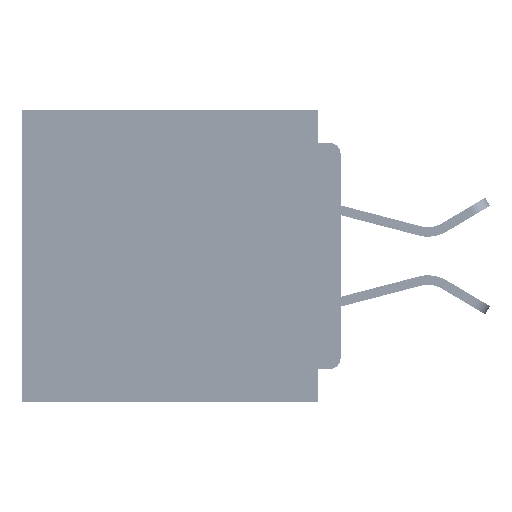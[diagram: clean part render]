
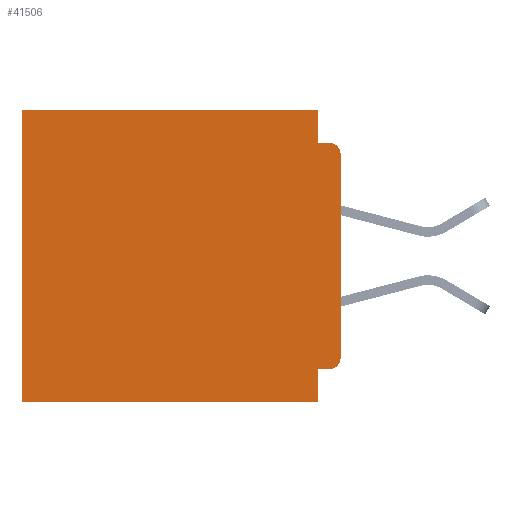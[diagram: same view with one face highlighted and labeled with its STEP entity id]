
A CAD part, left-side view. The second image highlights one B-rep face of the part: STEP entity #41506.
In plain terms, the highlighted planar face has unit normal (-1, 0, 0).
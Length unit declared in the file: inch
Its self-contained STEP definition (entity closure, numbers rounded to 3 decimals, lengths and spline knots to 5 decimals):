
#575 = CARTESIAN_POINT ( 'NONE',  ( 0.3, 0.015, -0.045 ) ) ;
#591 = DIRECTION ( 'NONE',  ( 0., 0., -1. ) ) ;
#2597 = EDGE_CURVE ( 'NONE', #43844, #50518, #33708, .T. ) ;
#2896 = LINE ( 'NONE', #24604, #13809 ) ;
#2907 = ORIENTED_EDGE ( 'NONE', *, *, #11951, .T. ) ;
#3120 = VECTOR ( 'NONE', #52583, 39.37008 ) ;
#3672 = ORIENTED_EDGE ( 'NONE', *, *, #30332, .F. ) ;
#3992 = CARTESIAN_POINT ( 'NONE',  ( 0.3, 0.015, -0.34 ) ) ;
#4407 = VERTEX_POINT ( 'NONE', #10277 ) ;
#4500 = CARTESIAN_POINT ( 'NONE',  ( 0.3, 0.015, -0.355 ) ) ;
#5869 = CARTESIAN_POINT ( 'NONE',  ( 0.3, 0., -0.34 ) ) ;
#5871 = EDGE_CURVE ( 'NONE', #4407, #50518, #24624, .T. ) ;
#6820 = AXIS2_PLACEMENT_3D ( 'NONE', #37404, #9763, #42036 ) ;
#6990 = CARTESIAN_POINT ( 'NONE',  ( 0.3, 0.031, -0.045 ) ) ;
#7002 = CARTESIAN_POINT ( 'NONE',  ( 0.3, 0.437, -0.4 ) ) ;
#7388 = PLANE ( 'NONE',  #40994 ) ;
#8461 = EDGE_CURVE ( 'NONE', #45742, #45604, #2896, .T. ) ;
#8656 = DIRECTION ( 'NONE',  ( 0., 0., -1. ) ) ;
#9176 = VECTOR ( 'NONE', #16141, 39.37008 ) ;
#9763 = DIRECTION ( 'NONE',  ( -1., 0., 0. ) ) ;
#10277 = CARTESIAN_POINT ( 'NONE',  ( 0.3, 0., -0.06 ) ) ;
#10694 = DIRECTION ( 'NONE',  ( 0., 1., 0. ) ) ;
#11133 = EDGE_CURVE ( 'NONE', #12591, #52123, #28607, .T. ) ;
#11951 = EDGE_CURVE ( 'NONE', #32054, #45604, #17674, .T. ) ;
#12055 = DIRECTION ( 'NONE',  ( 1., 0., 0. ) ) ;
#12591 = VERTEX_POINT ( 'NONE', #4500 ) ;
#13768 = LINE ( 'NONE', #38740, #3120 ) ;
#13809 = VECTOR ( 'NONE', #10694, 39.37008 ) ;
#14869 = ORIENTED_EDGE ( 'NONE', *, *, #21734, .F. ) ;
#16141 = DIRECTION ( 'NONE',  ( 0., -1., 0. ) ) ;
#16599 = CARTESIAN_POINT ( 'NONE',  ( 0.3, 0., -0.045 ) ) ;
#16727 = VECTOR ( 'NONE', #591, 39.37008 ) ;
#16891 = CIRCLE ( 'NONE', #19537, 0.015 ) ;
#17515 = CARTESIAN_POINT ( 'NONE',  ( 0.3, 0.031, -0.4 ) ) ;
#17674 = LINE ( 'NONE', #59514, #42197 ) ;
#17701 = ORIENTED_EDGE ( 'NONE', *, *, #5871, .T. ) ;
#18142 = LINE ( 'NONE', #42157, #16727 ) ;
#19439 = ORIENTED_EDGE ( 'NONE', *, *, #11133, .F. ) ;
#19537 = AXIS2_PLACEMENT_3D ( 'NONE', #3992, #36324, #8656 ) ;
#20912 = DIRECTION ( 'NONE',  ( 0., 1., 0. ) ) ;
#21206 = VERTEX_POINT ( 'NONE', #5869 ) ;
#21734 = EDGE_CURVE ( 'NONE', #4407, #21206, #44222, .T. ) ;
#22326 = LINE ( 'NONE', #57701, #33114 ) ;
#23179 = ORIENTED_EDGE ( 'NONE', *, *, #28295, .T. ) ;
#24604 = CARTESIAN_POINT ( 'NONE',  ( 0.3, 0., -0.4 ) ) ;
#24624 = CIRCLE ( 'NONE', #6820, 0.015 ) ;
#28295 = EDGE_CURVE ( 'NONE', #12591, #21206, #16891, .T. ) ;
#28607 = LINE ( 'NONE', #29842, #39431 ) ;
#29842 = CARTESIAN_POINT ( 'NONE',  ( 0.3, 0., -0.355 ) ) ;
#30332 = EDGE_CURVE ( 'NONE', #52123, #45742, #18142, .T. ) ;
#31114 = CARTESIAN_POINT ( 'NONE',  ( 0.3, 0.031, -0.355 ) ) ;
#31967 = VECTOR ( 'NONE', #46785, 39.37008 ) ;
#32054 = VERTEX_POINT ( 'NONE', #51603 ) ;
#32071 = DIRECTION ( 'NONE',  ( 0., 0., -1. ) ) ;
#33114 = VECTOR ( 'NONE', #20912, 39.37008 ) ;
#33708 = LINE ( 'NONE', #16599, #9176 ) ;
#34101 = EDGE_CURVE ( 'NONE', #42102, #43844, #13768, .T. ) ;
#34820 = EDGE_CURVE ( 'NONE', #42102, #32054, #22326, .T. ) ;
#36324 = DIRECTION ( 'NONE',  ( -1., 0., 0. ) ) ;
#37404 = CARTESIAN_POINT ( 'NONE',  ( 0.3, 0.015, -0.06 ) ) ;
#38740 = CARTESIAN_POINT ( 'NONE',  ( 0.3, 0.031, 0. ) ) ;
#39110 = DIRECTION ( 'NONE',  ( 0., 1., 0. ) ) ;
#39431 = VECTOR ( 'NONE', #39110, 39.37008 ) ;
#40689 = ORIENTED_EDGE ( 'NONE', *, *, #8461, .F. ) ;
#40752 = FACE_OUTER_BOUND ( 'NONE', #44073, .T. ) ;
#40994 = AXIS2_PLACEMENT_3D ( 'NONE', #48731, #12055, #44320 ) ;
#41506 = ADVANCED_FACE ( 'NONE', ( #40752 ), #7388, .F. ) ;
#42036 = DIRECTION ( 'NONE',  ( 0., 0., -1. ) ) ;
#42102 = VERTEX_POINT ( 'NONE', #57638 ) ;
#42157 = CARTESIAN_POINT ( 'NONE',  ( 0.3, 0.031, -0.4 ) ) ;
#42197 = VECTOR ( 'NONE', #32071, 39.37008 ) ;
#43844 = VERTEX_POINT ( 'NONE', #6990 ) ;
#44073 = EDGE_LOOP ( 'NONE', ( #14869, #17701, #47538, #55801, #44557, #2907, #40689, #3672, #19439, #23179 ) ) ;
#44222 = LINE ( 'NONE', #55762, #31967 ) ;
#44320 = DIRECTION ( 'NONE',  ( 0., 0., -1. ) ) ;
#44557 = ORIENTED_EDGE ( 'NONE', *, *, #34820, .T. ) ;
#45604 = VERTEX_POINT ( 'NONE', #7002 ) ;
#45742 = VERTEX_POINT ( 'NONE', #17515 ) ;
#46785 = DIRECTION ( 'NONE',  ( 0., 0., -1. ) ) ;
#47538 = ORIENTED_EDGE ( 'NONE', *, *, #2597, .F. ) ;
#48731 = CARTESIAN_POINT ( 'NONE',  ( 0.3, 0., -0.4 ) ) ;
#50518 = VERTEX_POINT ( 'NONE', #575 ) ;
#51603 = CARTESIAN_POINT ( 'NONE',  ( 0.3, 0.437, 0. ) ) ;
#52123 = VERTEX_POINT ( 'NONE', #31114 ) ;
#52583 = DIRECTION ( 'NONE',  ( 0., 0., -1. ) ) ;
#55762 = CARTESIAN_POINT ( 'NONE',  ( 0.3, 0., -0.4 ) ) ;
#55801 = ORIENTED_EDGE ( 'NONE', *, *, #34101, .F. ) ;
#57638 = CARTESIAN_POINT ( 'NONE',  ( 0.3, 0.031, 0. ) ) ;
#57701 = CARTESIAN_POINT ( 'NONE',  ( 0.3, 0., 0. ) ) ;
#59514 = CARTESIAN_POINT ( 'NONE',  ( 0.3, 0.437, -0.4 ) ) ;
